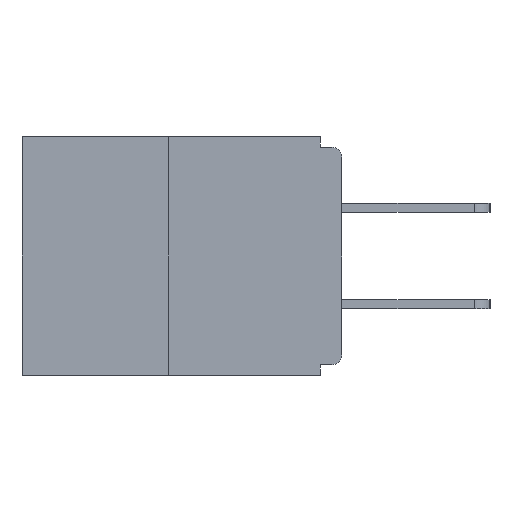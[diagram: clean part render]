
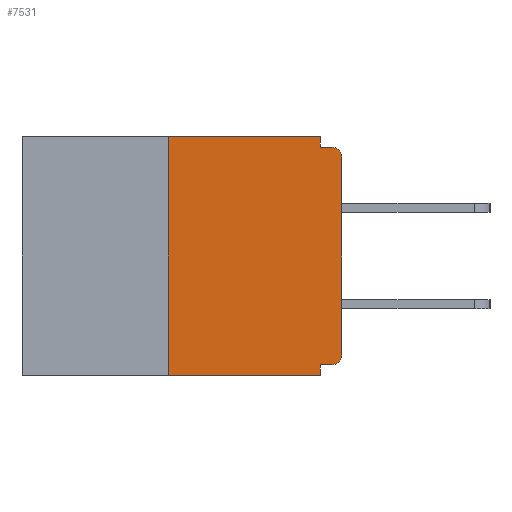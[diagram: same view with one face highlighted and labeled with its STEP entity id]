
A CAD part, left-side view. The second image highlights one B-rep face of the part: STEP entity #7531.
In plain terms, the highlighted planar face has unit normal (-1, 0, 0).
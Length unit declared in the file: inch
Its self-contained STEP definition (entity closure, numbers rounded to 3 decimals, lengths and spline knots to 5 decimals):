
#137 = EDGE_CURVE ( 'NONE', #19430, #411, #14718, .T. ) ;
#192 = LINE ( 'NONE', #1084, #18777 ) ;
#344 = CARTESIAN_POINT ( 'NONE',  ( 0., 0.25, 0. ) ) ;
#411 = VERTEX_POINT ( 'NONE', #19703 ) ;
#482 = LINE ( 'NONE', #12481, #7271 ) ;
#1019 = CARTESIAN_POINT ( 'NONE',  ( 0., 0.031, -0.328 ) ) ;
#1084 = CARTESIAN_POINT ( 'NONE',  ( 0., 0., -0.015 ) ) ;
#2182 = CARTESIAN_POINT ( 'NONE',  ( 0., 0.46, -0.343 ) ) ;
#3061 = DIRECTION ( 'NONE',  ( 0., 0., 1. ) ) ;
#3229 = DIRECTION ( 'NONE',  ( 0., 1., 0. ) ) ;
#3360 = ORIENTED_EDGE ( 'NONE', *, *, #22286, .F. ) ;
#3519 = VERTEX_POINT ( 'NONE', #10114 ) ;
#3702 = VECTOR ( 'NONE', #17305, 39.37008 ) ;
#3740 = VERTEX_POINT ( 'NONE', #23445 ) ;
#3899 = DIRECTION ( 'NONE',  ( 0., 0., -1. ) ) ;
#4554 = ORIENTED_EDGE ( 'NONE', *, *, #137, .F. ) ;
#4777 = CARTESIAN_POINT ( 'NONE',  ( 0., 0.015, -0.015 ) ) ;
#4846 = LINE ( 'NONE', #9484, #16624 ) ;
#5577 = DIRECTION ( 'NONE',  ( 0., 0., -1. ) ) ;
#7025 = DIRECTION ( 'NONE',  ( 1., 0., 0. ) ) ;
#7271 = VECTOR ( 'NONE', #3061, 39.37008 ) ;
#7531 = ADVANCED_FACE ( 'NONE', ( #27717 ), #23865, .F. ) ;
#8382 = CARTESIAN_POINT ( 'NONE',  ( 0., 0.031, -0.343 ) ) ;
#8662 = CARTESIAN_POINT ( 'NONE',  ( 0., 0.015, -0.313 ) ) ;
#9353 = VERTEX_POINT ( 'NONE', #4777 ) ;
#9390 = DIRECTION ( 'NONE',  ( 0., 0., -1. ) ) ;
#9484 = CARTESIAN_POINT ( 'NONE',  ( 0., 0.031, 0. ) ) ;
#9704 = CARTESIAN_POINT ( 'NONE',  ( 0., 0.46, 0. ) ) ;
#9899 = LINE ( 'NONE', #2182, #18989 ) ;
#10114 = CARTESIAN_POINT ( 'NONE',  ( 0., 0., -0.313 ) ) ;
#10908 = LINE ( 'NONE', #344, #3702 ) ;
#11510 = VECTOR ( 'NONE', #5577, 39.37008 ) ;
#12481 = CARTESIAN_POINT ( 'NONE',  ( 0., 0., 0. ) ) ;
#13484 = CARTESIAN_POINT ( 'NONE',  ( 0., 0.015, -0.03 ) ) ;
#13535 = VERTEX_POINT ( 'NONE', #1019 ) ;
#14103 = ORIENTED_EDGE ( 'NONE', *, *, #28998, .F. ) ;
#14138 = AXIS2_PLACEMENT_3D ( 'NONE', #23756, #7025, #9390 ) ;
#14718 = LINE ( 'NONE', #9704, #23425 ) ;
#15056 = VERTEX_POINT ( 'NONE', #22160 ) ;
#15149 = EDGE_CURVE ( 'NONE', #21013, #9353, #29378, .T. ) ;
#15204 = EDGE_CURVE ( 'NONE', #31064, #9353, #192, .T. ) ;
#15304 = LINE ( 'NONE', #8382, #11510 ) ;
#15558 = ORIENTED_EDGE ( 'NONE', *, *, #18860, .F. ) ;
#15739 = AXIS2_PLACEMENT_3D ( 'NONE', #13484, #20690, #18061 ) ;
#15890 = VERTEX_POINT ( 'NONE', #31115 ) ;
#16624 = VECTOR ( 'NONE', #26318, 39.37008 ) ;
#16652 = LINE ( 'NONE', #22598, #30649 ) ;
#16721 = EDGE_LOOP ( 'NONE', ( #4554, #14103, #20646, #27105, #3360, #28195, #23892, #23862, #24405, #15558 ) ) ;
#16820 = EDGE_CURVE ( 'NONE', #15890, #3519, #22425, .T. ) ;
#17305 = DIRECTION ( 'NONE',  ( 0., 0., 1. ) ) ;
#18061 = DIRECTION ( 'NONE',  ( 0., 0., -1. ) ) ;
#18777 = VECTOR ( 'NONE', #25323, 39.37008 ) ;
#18860 = EDGE_CURVE ( 'NONE', #411, #31064, #4846, .T. ) ;
#18935 = DIRECTION ( 'NONE',  ( 0., -1., 0. ) ) ;
#18989 = VECTOR ( 'NONE', #19464, 39.37008 ) ;
#19430 = VERTEX_POINT ( 'NONE', #22046 ) ;
#19464 = DIRECTION ( 'NONE',  ( 0., -1., 0. ) ) ;
#19703 = CARTESIAN_POINT ( 'NONE',  ( 0., 0.031, 0. ) ) ;
#20646 = ORIENTED_EDGE ( 'NONE', *, *, #27576, .T. ) ;
#20690 = DIRECTION ( 'NONE',  ( -1., 0., 0. ) ) ;
#20844 = AXIS2_PLACEMENT_3D ( 'NONE', #8662, #30808, #3899 ) ;
#21013 = VERTEX_POINT ( 'NONE', #25290 ) ;
#22046 = CARTESIAN_POINT ( 'NONE',  ( 0., 0.25, 0. ) ) ;
#22160 = CARTESIAN_POINT ( 'NONE',  ( 0., 0.031, -0.343 ) ) ;
#22286 = EDGE_CURVE ( 'NONE', #15890, #13535, #16652, .T. ) ;
#22425 = CIRCLE ( 'NONE', #20844, 0.015 ) ;
#22598 = CARTESIAN_POINT ( 'NONE',  ( 0., 0., -0.328 ) ) ;
#23425 = VECTOR ( 'NONE', #18935, 39.37008 ) ;
#23445 = CARTESIAN_POINT ( 'NONE',  ( 0., 0.25, -0.343 ) ) ;
#23756 = CARTESIAN_POINT ( 'NONE',  ( 0., 0.46, 0. ) ) ;
#23862 = ORIENTED_EDGE ( 'NONE', *, *, #15149, .T. ) ;
#23865 = PLANE ( 'NONE',  #14138 ) ;
#23892 = ORIENTED_EDGE ( 'NONE', *, *, #26112, .T. ) ;
#24405 = ORIENTED_EDGE ( 'NONE', *, *, #15204, .F. ) ;
#25290 = CARTESIAN_POINT ( 'NONE',  ( 0., 0., -0.03 ) ) ;
#25323 = DIRECTION ( 'NONE',  ( 0., -1., 0. ) ) ;
#25450 = EDGE_CURVE ( 'NONE', #13535, #15056, #15304, .T. ) ;
#26112 = EDGE_CURVE ( 'NONE', #3519, #21013, #482, .T. ) ;
#26318 = DIRECTION ( 'NONE',  ( 0., 0., -1. ) ) ;
#27105 = ORIENTED_EDGE ( 'NONE', *, *, #25450, .F. ) ;
#27576 = EDGE_CURVE ( 'NONE', #3740, #15056, #9899, .T. ) ;
#27717 = FACE_OUTER_BOUND ( 'NONE', #16721, .T. ) ;
#28195 = ORIENTED_EDGE ( 'NONE', *, *, #16820, .T. ) ;
#28987 = CARTESIAN_POINT ( 'NONE',  ( 0., 0.031, -0.015 ) ) ;
#28998 = EDGE_CURVE ( 'NONE', #3740, #19430, #10908, .T. ) ;
#29378 = CIRCLE ( 'NONE', #15739, 0.015 ) ;
#30649 = VECTOR ( 'NONE', #3229, 39.37008 ) ;
#30808 = DIRECTION ( 'NONE',  ( -1., 0., 0. ) ) ;
#31064 = VERTEX_POINT ( 'NONE', #28987 ) ;
#31115 = CARTESIAN_POINT ( 'NONE',  ( 0., 0.015, -0.328 ) ) ;
